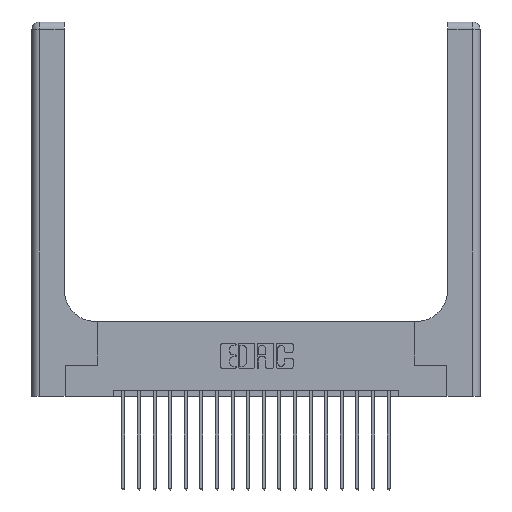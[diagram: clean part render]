
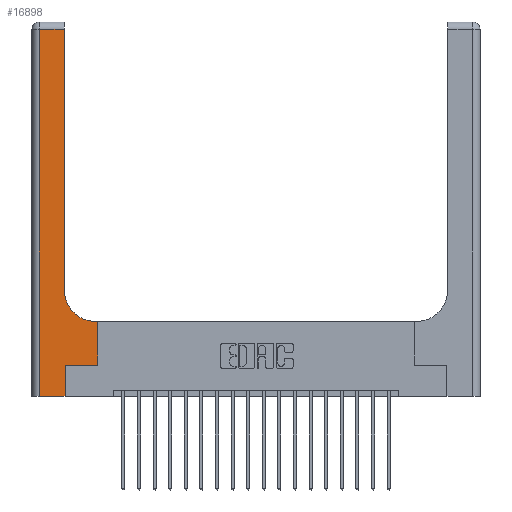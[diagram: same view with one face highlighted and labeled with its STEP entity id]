
A CAD part, top view. The second image highlights one B-rep face of the part: STEP entity #16898.
In plain terms, the highlighted planar face has unit normal (0, 0, 1).
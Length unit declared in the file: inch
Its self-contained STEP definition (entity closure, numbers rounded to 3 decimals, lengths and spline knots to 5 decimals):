
#60 = CARTESIAN_POINT ( 'NONE',  ( 0.26, 0.6, 0.37 ) ) ;
#71 = VECTOR ( 'NONE', #17560, 39.37008 ) ;
#204 = ORIENTED_EDGE ( 'NONE', *, *, #17139, .T. ) ;
#741 = EDGE_CURVE ( 'NONE', #13732, #12277, #4215, .T. ) ;
#805 = FACE_OUTER_BOUND ( 'NONE', #14863, .T. ) ;
#903 = PLANE ( 'NONE',  #12423 ) ;
#1500 = DIRECTION ( 'NONE',  ( 0., 1., 0. ) ) ;
#1506 = CARTESIAN_POINT ( 'NONE',  ( 0.528, 0.25, 0.37 ) ) ;
#1708 = DIRECTION ( 'NONE',  ( 0., 1., 0. ) ) ;
#1821 = EDGE_CURVE ( 'NONE', #9621, #12617, #12191, .T. ) ;
#2035 = ORIENTED_EDGE ( 'NONE', *, *, #741, .T. ) ;
#2669 = CARTESIAN_POINT ( 'NONE',  ( 0.265, 0., 0.37 ) ) ;
#2683 = DIRECTION ( 'NONE',  ( 0., 1., 0. ) ) ;
#3147 = EDGE_CURVE ( 'NONE', #12617, #5949, #19238, .T. ) ;
#3157 = CARTESIAN_POINT ( 'NONE',  ( 0.528, 0.6, 0.37 ) ) ;
#3362 = CARTESIAN_POINT ( 'NONE',  ( 0.26, 3., 0.37 ) ) ;
#3634 = EDGE_CURVE ( 'NONE', #12277, #14603, #11303, .T. ) ;
#3788 = AXIS2_PLACEMENT_3D ( 'NONE', #7108, #5531, #13457 ) ;
#4215 = LINE ( 'NONE', #10359, #18872 ) ;
#4675 = VECTOR ( 'NONE', #1500, 39.37008 ) ;
#5531 = DIRECTION ( 'NONE',  ( 0., 0., -1. ) ) ;
#5823 = DIRECTION ( 'NONE',  ( -1., 0., 0. ) ) ;
#5923 = CARTESIAN_POINT ( 'NONE',  ( 0., 3., 0.37 ) ) ;
#5949 = VERTEX_POINT ( 'NONE', #12043 ) ;
#6228 = DIRECTION ( 'NONE',  ( -1., 0., 0. ) ) ;
#7056 = ORIENTED_EDGE ( 'NONE', *, *, #18423, .T. ) ;
#7108 = CARTESIAN_POINT ( 'NONE',  ( 0.51, 0.85, 0.37 ) ) ;
#7401 = VECTOR ( 'NONE', #19294, 39.37008 ) ;
#7480 = CIRCLE ( 'NONE', #3788, 0.25 ) ;
#7493 = CARTESIAN_POINT ( 'NONE',  ( 0., 2.94, 0.37 ) ) ;
#9052 = CARTESIAN_POINT ( 'NONE',  ( 0.265, 0., 0.37 ) ) ;
#9198 = EDGE_CURVE ( 'NONE', #11136, #13732, #19813, .T. ) ;
#9299 = VECTOR ( 'NONE', #2683, 39.37008 ) ;
#9574 = CARTESIAN_POINT ( 'NONE',  ( 0.528, 0.25, 0.37 ) ) ;
#9621 = VERTEX_POINT ( 'NONE', #14835 ) ;
#10256 = VERTEX_POINT ( 'NONE', #14181 ) ;
#10359 = CARTESIAN_POINT ( 'NONE',  ( 0.265, 0.25, 0.37 ) ) ;
#11136 = VERTEX_POINT ( 'NONE', #2669 ) ;
#11226 = LINE ( 'NONE', #60, #71 ) ;
#11275 = CARTESIAN_POINT ( 'NONE',  ( 0., 0., 0.37 ) ) ;
#11303 = LINE ( 'NONE', #1506, #20152 ) ;
#11429 = CARTESIAN_POINT ( 'NONE',  ( 0.06, 3., 0.37 ) ) ;
#12015 = ORIENTED_EDGE ( 'NONE', *, *, #14542, .T. ) ;
#12043 = CARTESIAN_POINT ( 'NONE',  ( 0.06, 0., 0.37 ) ) ;
#12191 = LINE ( 'NONE', #7493, #12451 ) ;
#12277 = VERTEX_POINT ( 'NONE', #9574 ) ;
#12298 = DIRECTION ( 'NONE',  ( 0., 0., -1. ) ) ;
#12423 = AXIS2_PLACEMENT_3D ( 'NONE', #5923, #12298, #5823 ) ;
#12451 = VECTOR ( 'NONE', #6228, 39.37008 ) ;
#12617 = VERTEX_POINT ( 'NONE', #18920 ) ;
#12930 = VERTEX_POINT ( 'NONE', #20064 ) ;
#13094 = DIRECTION ( 'NONE',  ( 0., -1., 0. ) ) ;
#13457 = DIRECTION ( 'NONE',  ( 1., 0., 0. ) ) ;
#13732 = VERTEX_POINT ( 'NONE', #14566 ) ;
#14181 = CARTESIAN_POINT ( 'NONE',  ( 0.51, 0.6, 0.37 ) ) ;
#14197 = LINE ( 'NONE', #11275, #7401 ) ;
#14314 = LINE ( 'NONE', #3362, #4675 ) ;
#14520 = VECTOR ( 'NONE', #13094, 39.37008 ) ;
#14542 = EDGE_CURVE ( 'NONE', #12930, #9621, #14314, .T. ) ;
#14566 = CARTESIAN_POINT ( 'NONE',  ( 0.265, 0.25, 0.37 ) ) ;
#14603 = VERTEX_POINT ( 'NONE', #3157 ) ;
#14835 = CARTESIAN_POINT ( 'NONE',  ( 0.26, 2.94, 0.37 ) ) ;
#14863 = EDGE_LOOP ( 'NONE', ( #12015, #17725, #20047, #19944, #20246, #2035, #15571, #204, #7056 ) ) ;
#14949 = DIRECTION ( 'NONE',  ( 1., 0., 0. ) ) ;
#15571 = ORIENTED_EDGE ( 'NONE', *, *, #3634, .T. ) ;
#16255 = EDGE_CURVE ( 'NONE', #5949, #11136, #14197, .T. ) ;
#16898 = ADVANCED_FACE ( 'NONE', ( #805 ), #903, .F. ) ;
#17139 = EDGE_CURVE ( 'NONE', #14603, #10256, #11226, .T. ) ;
#17560 = DIRECTION ( 'NONE',  ( -1., 0., 0. ) ) ;
#17725 = ORIENTED_EDGE ( 'NONE', *, *, #1821, .T. ) ;
#18423 = EDGE_CURVE ( 'NONE', #10256, #12930, #7480, .T. ) ;
#18872 = VECTOR ( 'NONE', #14949, 39.37008 ) ;
#18920 = CARTESIAN_POINT ( 'NONE',  ( 0.06, 2.94, 0.37 ) ) ;
#19238 = LINE ( 'NONE', #11429, #14520 ) ;
#19294 = DIRECTION ( 'NONE',  ( 1., 0., 0. ) ) ;
#19813 = LINE ( 'NONE', #9052, #9299 ) ;
#19944 = ORIENTED_EDGE ( 'NONE', *, *, #16255, .T. ) ;
#20047 = ORIENTED_EDGE ( 'NONE', *, *, #3147, .T. ) ;
#20064 = CARTESIAN_POINT ( 'NONE',  ( 0.26, 0.85, 0.37 ) ) ;
#20152 = VECTOR ( 'NONE', #1708, 39.37008 ) ;
#20246 = ORIENTED_EDGE ( 'NONE', *, *, #9198, .T. ) ;
